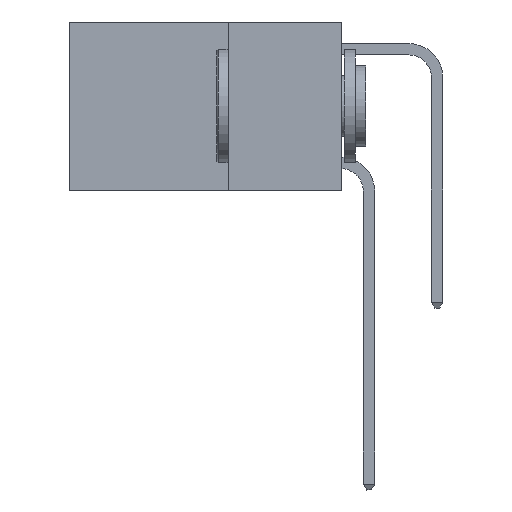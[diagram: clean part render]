
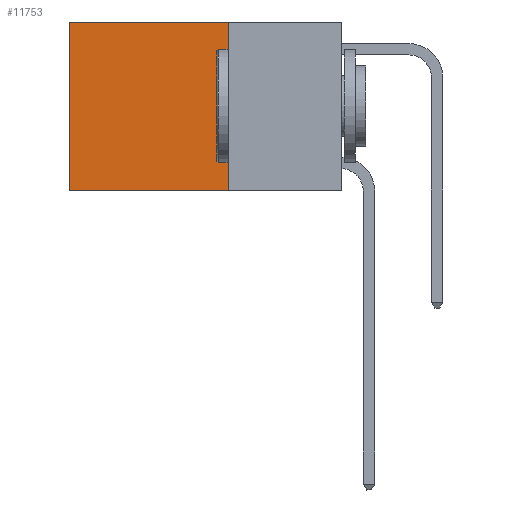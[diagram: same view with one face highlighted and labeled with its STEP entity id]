
A CAD part, left-side view. The second image highlights one B-rep face of the part: STEP entity #11753.
In plain terms, the highlighted planar face has unit normal (-1, 0, 0).
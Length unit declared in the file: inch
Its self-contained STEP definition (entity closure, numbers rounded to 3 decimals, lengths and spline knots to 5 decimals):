
#1062 = CARTESIAN_POINT ( 'NONE',  ( 0.2625, 0.25, 0. ) ) ;
#1468 = AXIS2_PLACEMENT_3D ( 'NONE', #12324, #9924, #17341 ) ;
#1490 = EDGE_CURVE ( 'NONE', #4059, #3297, #1640, .T. ) ;
#1640 = LINE ( 'NONE', #7596, #17405 ) ;
#2650 = DIRECTION ( 'NONE',  ( 0., 0., -1. ) ) ;
#3297 = VERTEX_POINT ( 'NONE', #15970 ) ;
#4059 = VERTEX_POINT ( 'NONE', #5791 ) ;
#4077 = DIRECTION ( 'NONE',  ( 0., 0., -1. ) ) ;
#5791 = CARTESIAN_POINT ( 'NONE',  ( 0.2625, 0.25, 0. ) ) ;
#6092 = VECTOR ( 'NONE', #19693, 39.37008 ) ;
#6326 = ORIENTED_EDGE ( 'NONE', *, *, #1490, .T. ) ;
#6442 = ORIENTED_EDGE ( 'NONE', *, *, #18641, .F. ) ;
#7596 = CARTESIAN_POINT ( 'NONE',  ( 0.2625, 0.25, 0. ) ) ;
#8619 = ORIENTED_EDGE ( 'NONE', *, *, #13361, .T. ) ;
#8963 = LINE ( 'NONE', #23596, #6092 ) ;
#9363 = EDGE_CURVE ( 'NONE', #4059, #12385, #23245, .T. ) ;
#9924 = DIRECTION ( 'NONE',  ( 1., 0., 0. ) ) ;
#11753 = ADVANCED_FACE ( 'NONE', ( #21475 ), #12091, .F. ) ;
#11779 = VERTEX_POINT ( 'NONE', #17696 ) ;
#12091 = PLANE ( 'NONE',  #1468 ) ;
#12324 = CARTESIAN_POINT ( 'NONE',  ( 0.2625, 0.25, 0. ) ) ;
#12385 = VERTEX_POINT ( 'NONE', #15207 ) ;
#13361 = EDGE_CURVE ( 'NONE', #3297, #11779, #19407, .T. ) ;
#15207 = CARTESIAN_POINT ( 'NONE',  ( 0.2625, 0.25, -0.37 ) ) ;
#15970 = CARTESIAN_POINT ( 'NONE',  ( 0.2625, 0.6, 0. ) ) ;
#16069 = VECTOR ( 'NONE', #4077, 39.37008 ) ;
#17341 = DIRECTION ( 'NONE',  ( 0., 0., -1. ) ) ;
#17368 = ORIENTED_EDGE ( 'NONE', *, *, #9363, .F. ) ;
#17405 = VECTOR ( 'NONE', #24058, 39.37008 ) ;
#17696 = CARTESIAN_POINT ( 'NONE',  ( 0.2625, 0.6, -0.37 ) ) ;
#18641 = EDGE_CURVE ( 'NONE', #12385, #11779, #8963, .T. ) ;
#19407 = LINE ( 'NONE', #20889, #16069 ) ;
#19693 = DIRECTION ( 'NONE',  ( 0., 1., 0. ) ) ;
#20589 = EDGE_LOOP ( 'NONE', ( #8619, #6442, #17368, #6326 ) ) ;
#20889 = CARTESIAN_POINT ( 'NONE',  ( 0.2625, 0.6, 0. ) ) ;
#21475 = FACE_OUTER_BOUND ( 'NONE', #20589, .T. ) ;
#23059 = VECTOR ( 'NONE', #2650, 39.37008 ) ;
#23245 = LINE ( 'NONE', #1062, #23059 ) ;
#23596 = CARTESIAN_POINT ( 'NONE',  ( 0.2625, 0.25, -0.37 ) ) ;
#24058 = DIRECTION ( 'NONE',  ( 0., 1., 0. ) ) ;
